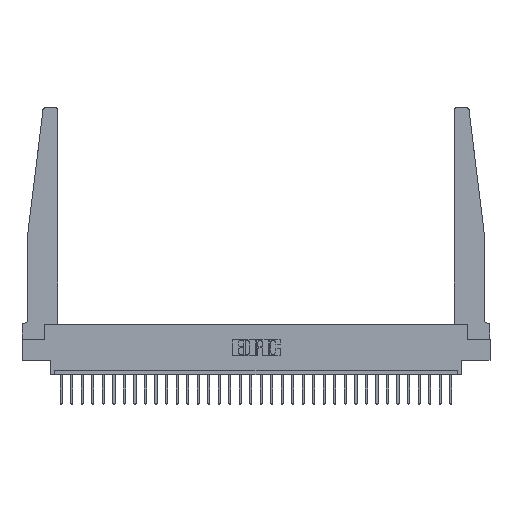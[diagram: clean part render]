
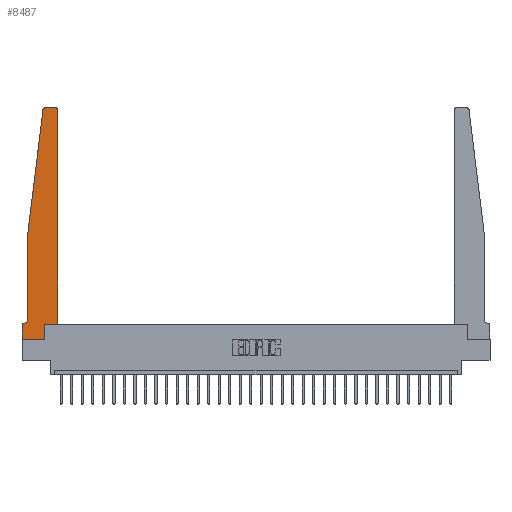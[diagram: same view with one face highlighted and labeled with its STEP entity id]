
A CAD part, top view. The second image highlights one B-rep face of the part: STEP entity #8487.
In plain terms, the highlighted planar face has unit normal (0, 0, 1).
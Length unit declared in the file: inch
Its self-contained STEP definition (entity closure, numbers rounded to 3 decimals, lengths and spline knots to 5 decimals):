
#104 = VERTEX_POINT ( 'NONE', #26947 ) ;
#134 = VERTEX_POINT ( 'NONE', #1740 ) ;
#159 = DIRECTION ( 'NONE',  ( -1., 0., 0. ) ) ;
#182 = ORIENTED_EDGE ( 'NONE', *, *, #25035, .T. ) ;
#1265 = DIRECTION ( 'NONE',  ( -1., 0., 0. ) ) ;
#1653 = CARTESIAN_POINT ( 'NONE',  ( 0.395, 2.72, 0.37 ) ) ;
#1740 = CARTESIAN_POINT ( 'NONE',  ( 0.27653, 2.75, 0.37 ) ) ;
#1869 = VERTEX_POINT ( 'NONE', #10354 ) ;
#2063 = LINE ( 'NONE', #12593, #19301 ) ;
#2407 = CARTESIAN_POINT ( 'NONE',  ( 0.065, 1.25, 0.37 ) ) ;
#2443 = ORIENTED_EDGE ( 'NONE', *, *, #19923, .T. ) ;
#3105 = VERTEX_POINT ( 'NONE', #11885 ) ;
#3293 = LINE ( 'NONE', #21698, #3986 ) ;
#3359 = VERTEX_POINT ( 'NONE', #9761 ) ;
#3549 = CARTESIAN_POINT ( 'NONE',  ( 0., 0., 0.37 ) ) ;
#3667 = ORIENTED_EDGE ( 'NONE', *, *, #25597, .T. ) ;
#3986 = VECTOR ( 'NONE', #1265, 39.37008 ) ;
#4002 = ORIENTED_EDGE ( 'NONE', *, *, #8901, .T. ) ;
#4023 = LINE ( 'NONE', #13190, #5443 ) ;
#4463 = VERTEX_POINT ( 'NONE', #25299 ) ;
#5429 = AXIS2_PLACEMENT_3D ( 'NONE', #1653, #24328, #8838 ) ;
#5443 = VECTOR ( 'NONE', #19859, 39.37008 ) ;
#5511 = EDGE_CURVE ( 'NONE', #26714, #8507, #23705, .T. ) ;
#5686 = EDGE_CURVE ( 'NONE', #1869, #4463, #20733, .T. ) ;
#5876 = CARTESIAN_POINT ( 'NONE',  ( 0.425, 2.72, 0.37 ) ) ;
#6259 = DIRECTION ( 'NONE',  ( 0., 0., 1. ) ) ;
#6863 = VECTOR ( 'NONE', #28720, 39.37008 ) ;
#6899 = CARTESIAN_POINT ( 'NONE',  ( 0., 0.1875, 0.37 ) ) ;
#6936 = DIRECTION ( 'NONE',  ( 0., -1., 0. ) ) ;
#8069 = ORIENTED_EDGE ( 'NONE', *, *, #5686, .T. ) ;
#8423 = DIRECTION ( 'NONE',  ( 1., 0., 0. ) ) ;
#8487 = ADVANCED_FACE ( 'NONE', ( #15712 ), #11330, .T. ) ;
#8507 = VERTEX_POINT ( 'NONE', #13788 ) ;
#8838 = DIRECTION ( 'NONE',  ( 1., 0., 0. ) ) ;
#8901 = EDGE_CURVE ( 'NONE', #23934, #26194, #28233, .T. ) ;
#9005 = VECTOR ( 'NONE', #9323, 39.37008 ) ;
#9323 = DIRECTION ( 'NONE',  ( -0.122, -0.992, 0. ) ) ;
#9761 = CARTESIAN_POINT ( 'NONE',  ( 0.425, 0.18, 0.37 ) ) ;
#10354 = CARTESIAN_POINT ( 'NONE',  ( 0., 0.1875, 0.37 ) ) ;
#10697 = ORIENTED_EDGE ( 'NONE', *, *, #28764, .T. ) ;
#10744 = CARTESIAN_POINT ( 'NONE',  ( 0.065, 0.2375, 0.37 ) ) ;
#11279 = DIRECTION ( 'NONE',  ( 0., -1., 0. ) ) ;
#11330 = PLANE ( 'NONE',  #21880 ) ;
#11885 = CARTESIAN_POINT ( 'NONE',  ( 0.2605, 0.18, 0.37 ) ) ;
#12421 = CARTESIAN_POINT ( 'NONE',  ( 0.2605, 0., 0.37 ) ) ;
#12593 = CARTESIAN_POINT ( 'NONE',  ( 0.425, 0.18, 0.37 ) ) ;
#13190 = CARTESIAN_POINT ( 'NONE',  ( 0.2605, 0.18, 0.37 ) ) ;
#13788 = CARTESIAN_POINT ( 'NONE',  ( 0.395, 2.75, 0.37 ) ) ;
#13996 = VECTOR ( 'NONE', #17202, 39.37008 ) ;
#14367 = ORIENTED_EDGE ( 'NONE', *, *, #28911, .T. ) ;
#14698 = LINE ( 'NONE', #28839, #25865 ) ;
#14869 = DIRECTION ( 'NONE',  ( 0., 1., 0. ) ) ;
#15134 = ORIENTED_EDGE ( 'NONE', *, *, #15856, .T. ) ;
#15189 = CARTESIAN_POINT ( 'NONE',  ( 0., 0., 0.37 ) ) ;
#15254 = AXIS2_PLACEMENT_3D ( 'NONE', #15330, #6259, #8423 ) ;
#15330 = CARTESIAN_POINT ( 'NONE',  ( 0.27653, 2.72, 0.37 ) ) ;
#15712 = FACE_OUTER_BOUND ( 'NONE', #23372, .T. ) ;
#15856 = EDGE_CURVE ( 'NONE', #26194, #1869, #21347, .T. ) ;
#15975 = LINE ( 'NONE', #2407, #16331 ) ;
#16038 = ORIENTED_EDGE ( 'NONE', *, *, #22831, .T. ) ;
#16078 = LINE ( 'NONE', #16208, #9005 ) ;
#16208 = CARTESIAN_POINT ( 'NONE',  ( 0.065, 1.25, 0.37 ) ) ;
#16331 = VECTOR ( 'NONE', #11279, 39.37008 ) ;
#16501 = EDGE_CURVE ( 'NONE', #3105, #3359, #14698, .T. ) ;
#16523 = ORIENTED_EDGE ( 'NONE', *, *, #5511, .T. ) ;
#17202 = DIRECTION ( 'NONE',  ( -1., 0., 0. ) ) ;
#18363 = VERTEX_POINT ( 'NONE', #28659 ) ;
#18804 = LINE ( 'NONE', #15189, #6863 ) ;
#19301 = VECTOR ( 'NONE', #14869, 39.37008 ) ;
#19612 = CIRCLE ( 'NONE', #15254, 0.03 ) ;
#19859 = DIRECTION ( 'NONE',  ( 0., 1., 0. ) ) ;
#19923 = EDGE_CURVE ( 'NONE', #8507, #134, #3293, .T. ) ;
#20301 = DIRECTION ( 'NONE',  ( 0., 0., -1. ) ) ;
#20733 = LINE ( 'NONE', #3549, #26654 ) ;
#21347 = LINE ( 'NONE', #26072, #13996 ) ;
#21698 = CARTESIAN_POINT ( 'NONE',  ( 0.25, 2.75, 0.37 ) ) ;
#21880 = AXIS2_PLACEMENT_3D ( 'NONE', #6899, #22692, #27155 ) ;
#22455 = CARTESIAN_POINT ( 'NONE',  ( 0.015, 0.2375, 0.37 ) ) ;
#22692 = DIRECTION ( 'NONE',  ( 0., 0., 1. ) ) ;
#22823 = DIRECTION ( 'NONE',  ( 1., 0., 0. ) ) ;
#22831 = EDGE_CURVE ( 'NONE', #134, #18363, #19612, .T. ) ;
#23372 = EDGE_LOOP ( 'NONE', ( #2443, #16038, #27141, #14367, #4002, #15134, #8069, #10697, #182, #27151, #3667, #16523 ) ) ;
#23388 = AXIS2_PLACEMENT_3D ( 'NONE', #22455, #20301, #159 ) ;
#23705 = CIRCLE ( 'NONE', #5429, 0.03 ) ;
#23934 = VERTEX_POINT ( 'NONE', #10744 ) ;
#24231 = EDGE_CURVE ( 'NONE', #18363, #104, #16078, .T. ) ;
#24328 = DIRECTION ( 'NONE',  ( 0., 0., 1. ) ) ;
#25035 = EDGE_CURVE ( 'NONE', #28580, #3105, #4023, .T. ) ;
#25299 = CARTESIAN_POINT ( 'NONE',  ( 0., 0., 0.37 ) ) ;
#25597 = EDGE_CURVE ( 'NONE', #3359, #26714, #2063, .T. ) ;
#25865 = VECTOR ( 'NONE', #22823, 39.37008 ) ;
#26072 = CARTESIAN_POINT ( 'NONE',  ( 0.065, 0.1875, 0.37 ) ) ;
#26194 = VERTEX_POINT ( 'NONE', #26698 ) ;
#26654 = VECTOR ( 'NONE', #6936, 39.37008 ) ;
#26698 = CARTESIAN_POINT ( 'NONE',  ( 0.015, 0.1875, 0.37 ) ) ;
#26714 = VERTEX_POINT ( 'NONE', #5876 ) ;
#26947 = CARTESIAN_POINT ( 'NONE',  ( 0.065, 1.25, 0.37 ) ) ;
#27141 = ORIENTED_EDGE ( 'NONE', *, *, #24231, .T. ) ;
#27151 = ORIENTED_EDGE ( 'NONE', *, *, #16501, .T. ) ;
#27155 = DIRECTION ( 'NONE',  ( 1., 0., 0. ) ) ;
#28233 = CIRCLE ( 'NONE', #23388, 0.05 ) ;
#28580 = VERTEX_POINT ( 'NONE', #12421 ) ;
#28659 = CARTESIAN_POINT ( 'NONE',  ( 0.24675, 2.72367, 0.37 ) ) ;
#28720 = DIRECTION ( 'NONE',  ( 1., 0., 0. ) ) ;
#28764 = EDGE_CURVE ( 'NONE', #4463, #28580, #18804, .T. ) ;
#28839 = CARTESIAN_POINT ( 'NONE',  ( 0.425, 0.18, 0.37 ) ) ;
#28911 = EDGE_CURVE ( 'NONE', #104, #23934, #15975, .T. ) ;
